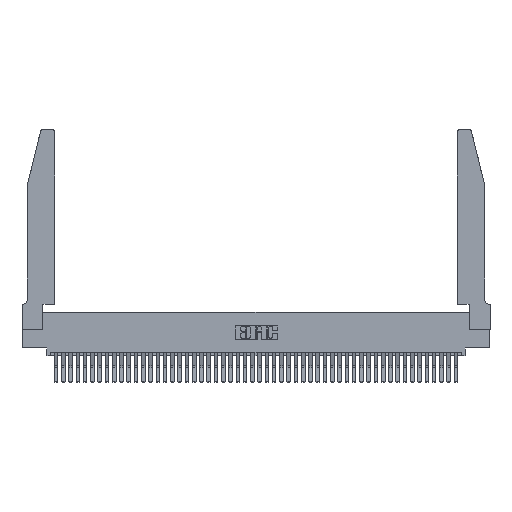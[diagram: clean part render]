
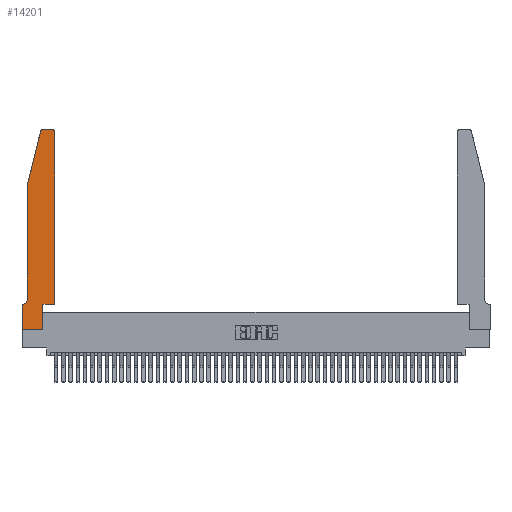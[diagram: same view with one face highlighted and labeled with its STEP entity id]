
A CAD part, top view. The second image highlights one B-rep face of the part: STEP entity #14201.
In plain terms, the highlighted planar face has unit normal (0, 0, 1).
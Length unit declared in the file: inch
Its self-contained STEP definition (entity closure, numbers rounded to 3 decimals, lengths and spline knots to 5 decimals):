
#163 = DIRECTION ( 'NONE',  ( 0., 0., 1. ) ) ;
#450 = VECTOR ( 'NONE', #40606, 39.37008 ) ;
#716 = ORIENTED_EDGE ( 'NONE', *, *, #17421, .T. ) ;
#1176 = VECTOR ( 'NONE', #37125, 39.37008 ) ;
#1882 = VERTEX_POINT ( 'NONE', #31213 ) ;
#2322 = FACE_OUTER_BOUND ( 'NONE', #12384, .T. ) ;
#2471 = EDGE_CURVE ( 'NONE', #14342, #13260, #43008, .T. ) ;
#4183 = CARTESIAN_POINT ( 'NONE',  ( 0.0055, 0.42, 0.37 ) ) ;
#4243 = CARTESIAN_POINT ( 'NONE',  ( 0.0755, 2., 0.37 ) ) ;
#5620 = VERTEX_POINT ( 'NONE', #10899 ) ;
#5665 = CARTESIAN_POINT ( 'NONE',  ( 0.0755, 2., 0.37 ) ) ;
#6122 = LINE ( 'NONE', #32984, #24334 ) ;
#6371 = EDGE_CURVE ( 'NONE', #27313, #14342, #20022, .T. ) ;
#6618 = DIRECTION ( 'NONE',  ( 1., 0., 0. ) ) ;
#7931 = DIRECTION ( 'NONE',  ( -1., 0., 0. ) ) ;
#8810 = ORIENTED_EDGE ( 'NONE', *, *, #24185, .T. ) ;
#8826 = AXIS2_PLACEMENT_3D ( 'NONE', #31374, #35017, #13395 ) ;
#9985 = LINE ( 'NONE', #10367, #37688 ) ;
#10309 = LINE ( 'NONE', #18974, #450 ) ;
#10367 = CARTESIAN_POINT ( 'NONE',  ( 0.4505, 0.35, 0.37 ) ) ;
#10899 = CARTESIAN_POINT ( 'NONE',  ( 0.25487, 2.72718, 0.37 ) ) ;
#12384 = EDGE_LOOP ( 'NONE', ( #39900, #14503, #35956, #38228, #39353, #23552, #8810, #43355, #44497, #716, #32048, #46213 ) ) ;
#13260 = VERTEX_POINT ( 'NONE', #17899 ) ;
#13395 = DIRECTION ( 'NONE',  ( 1., 0., 0. ) ) ;
#14201 = ADVANCED_FACE ( 'NONE', ( #2322 ), #31214, .T. ) ;
#14342 = VERTEX_POINT ( 'NONE', #39270 ) ;
#14469 = EDGE_CURVE ( 'NONE', #26874, #27042, #21202, .T. ) ;
#14503 = ORIENTED_EDGE ( 'NONE', *, *, #39958, .T. ) ;
#14711 = AXIS2_PLACEMENT_3D ( 'NONE', #22064, #163, #25683 ) ;
#15624 = CARTESIAN_POINT ( 'NONE',  ( 0., 0., 0.37 ) ) ;
#16145 = DIRECTION ( 'NONE',  ( 0., 1., 0. ) ) ;
#16311 = CARTESIAN_POINT ( 'NONE',  ( 0.2865, 0., 0.37 ) ) ;
#16578 = DIRECTION ( 'NONE',  ( 0., -1., 0. ) ) ;
#16744 = VECTOR ( 'NONE', #21218, 39.37008 ) ;
#17421 = EDGE_CURVE ( 'NONE', #39728, #44585, #9985, .T. ) ;
#17598 = CARTESIAN_POINT ( 'NONE',  ( 0., 0., 0.37 ) ) ;
#17899 = CARTESIAN_POINT ( 'NONE',  ( 0., 0.35, 0.37 ) ) ;
#18279 = EDGE_CURVE ( 'NONE', #27042, #1882, #39863, .T. ) ;
#18412 = DIRECTION ( 'NONE',  ( 0., 0., 1. ) ) ;
#18974 = CARTESIAN_POINT ( 'NONE',  ( 0.2865, 0.35, 0.37 ) ) ;
#19801 = CARTESIAN_POINT ( 'NONE',  ( 0.0755, 0.35, 0.37 ) ) ;
#20022 = CIRCLE ( 'NONE', #24083, 0.07 ) ;
#21202 = CIRCLE ( 'NONE', #42776, 0.03 ) ;
#21218 = DIRECTION ( 'NONE',  ( 0., -1., 0. ) ) ;
#21223 = CARTESIAN_POINT ( 'NONE',  ( 0.2865, 0.35, 0.37 ) ) ;
#21336 = VECTOR ( 'NONE', #16145, 39.37008 ) ;
#22064 = CARTESIAN_POINT ( 'NONE',  ( 0.284, 2.72, 0.37 ) ) ;
#22278 = DIRECTION ( 'NONE',  ( -0.239, -0.971, 0. ) ) ;
#22717 = EDGE_CURVE ( 'NONE', #44585, #26874, #30926, .T. ) ;
#22774 = CARTESIAN_POINT ( 'NONE',  ( 0.2605, 2.75, 0.37 ) ) ;
#23459 = DIRECTION ( 'NONE',  ( -1., 0., 0. ) ) ;
#23552 = ORIENTED_EDGE ( 'NONE', *, *, #2471, .T. ) ;
#24083 = AXIS2_PLACEMENT_3D ( 'NONE', #4183, #29636, #7931 ) ;
#24185 = EDGE_CURVE ( 'NONE', #13260, #40531, #26341, .T. ) ;
#24334 = VECTOR ( 'NONE', #22278, 39.37008 ) ;
#25683 = DIRECTION ( 'NONE',  ( 1., 0., 0. ) ) ;
#25724 = EDGE_CURVE ( 'NONE', #41271, #27313, #33530, .T. ) ;
#25778 = VECTOR ( 'NONE', #33595, 39.37008 ) ;
#25798 = CARTESIAN_POINT ( 'NONE',  ( 0., 0., 0.37 ) ) ;
#26341 = LINE ( 'NONE', #17598, #16744 ) ;
#26874 = VERTEX_POINT ( 'NONE', #44258 ) ;
#27042 = VERTEX_POINT ( 'NONE', #41398 ) ;
#27053 = VERTEX_POINT ( 'NONE', #16311 ) ;
#27313 = VERTEX_POINT ( 'NONE', #39324 ) ;
#29636 = DIRECTION ( 'NONE',  ( 0., 0., -1. ) ) ;
#30397 = EDGE_CURVE ( 'NONE', #5620, #41271, #6122, .T. ) ;
#30926 = LINE ( 'NONE', #34115, #21336 ) ;
#31213 = CARTESIAN_POINT ( 'NONE',  ( 0.284, 2.75, 0.37 ) ) ;
#31214 = PLANE ( 'NONE',  #8826 ) ;
#31265 = VECTOR ( 'NONE', #16578, 39.37008 ) ;
#31374 = CARTESIAN_POINT ( 'NONE',  ( 0., 0.35, 0.37 ) ) ;
#32048 = ORIENTED_EDGE ( 'NONE', *, *, #22717, .T. ) ;
#32984 = CARTESIAN_POINT ( 'NONE',  ( 0.0755, 2., 0.37 ) ) ;
#33530 = LINE ( 'NONE', #5665, #31265 ) ;
#33595 = DIRECTION ( 'NONE',  ( 1., 0., 0. ) ) ;
#34115 = CARTESIAN_POINT ( 'NONE',  ( 0.4505, 0.35, 0.37 ) ) ;
#35017 = DIRECTION ( 'NONE',  ( 0., 0., 1. ) ) ;
#35396 = LINE ( 'NONE', #15624, #25778 ) ;
#35956 = ORIENTED_EDGE ( 'NONE', *, *, #30397, .T. ) ;
#37125 = DIRECTION ( 'NONE',  ( -1., 0., 0. ) ) ;
#37688 = VECTOR ( 'NONE', #6618, 39.37008 ) ;
#38228 = ORIENTED_EDGE ( 'NONE', *, *, #25724, .T. ) ;
#38863 = EDGE_CURVE ( 'NONE', #40531, #27053, #35396, .T. ) ;
#39270 = CARTESIAN_POINT ( 'NONE',  ( 0.0055, 0.35, 0.37 ) ) ;
#39324 = CARTESIAN_POINT ( 'NONE',  ( 0.0755, 0.42, 0.37 ) ) ;
#39353 = ORIENTED_EDGE ( 'NONE', *, *, #6371, .T. ) ;
#39728 = VERTEX_POINT ( 'NONE', #21223 ) ;
#39863 = LINE ( 'NONE', #22774, #1176 ) ;
#39900 = ORIENTED_EDGE ( 'NONE', *, *, #18279, .T. ) ;
#39958 = EDGE_CURVE ( 'NONE', #1882, #5620, #45455, .T. ) ;
#40053 = CARTESIAN_POINT ( 'NONE',  ( 0.4205, 2.72, 0.37 ) ) ;
#40531 = VERTEX_POINT ( 'NONE', #25798 ) ;
#40606 = DIRECTION ( 'NONE',  ( 0., 1., 0. ) ) ;
#41271 = VERTEX_POINT ( 'NONE', #4243 ) ;
#41398 = CARTESIAN_POINT ( 'NONE',  ( 0.4205, 2.75, 0.37 ) ) ;
#41867 = VECTOR ( 'NONE', #23459, 39.37008 ) ;
#42776 = AXIS2_PLACEMENT_3D ( 'NONE', #40053, #18412, #43685 ) ;
#42836 = CARTESIAN_POINT ( 'NONE',  ( 0.4505, 0.35, 0.37 ) ) ;
#43008 = LINE ( 'NONE', #19801, #41867 ) ;
#43355 = ORIENTED_EDGE ( 'NONE', *, *, #38863, .T. ) ;
#43685 = DIRECTION ( 'NONE',  ( 1., 0., 0. ) ) ;
#44258 = CARTESIAN_POINT ( 'NONE',  ( 0.4505, 2.72, 0.37 ) ) ;
#44497 = ORIENTED_EDGE ( 'NONE', *, *, #46242, .T. ) ;
#44585 = VERTEX_POINT ( 'NONE', #42836 ) ;
#45455 = CIRCLE ( 'NONE', #14711, 0.03 ) ;
#46213 = ORIENTED_EDGE ( 'NONE', *, *, #14469, .T. ) ;
#46242 = EDGE_CURVE ( 'NONE', #27053, #39728, #10309, .T. ) ;
